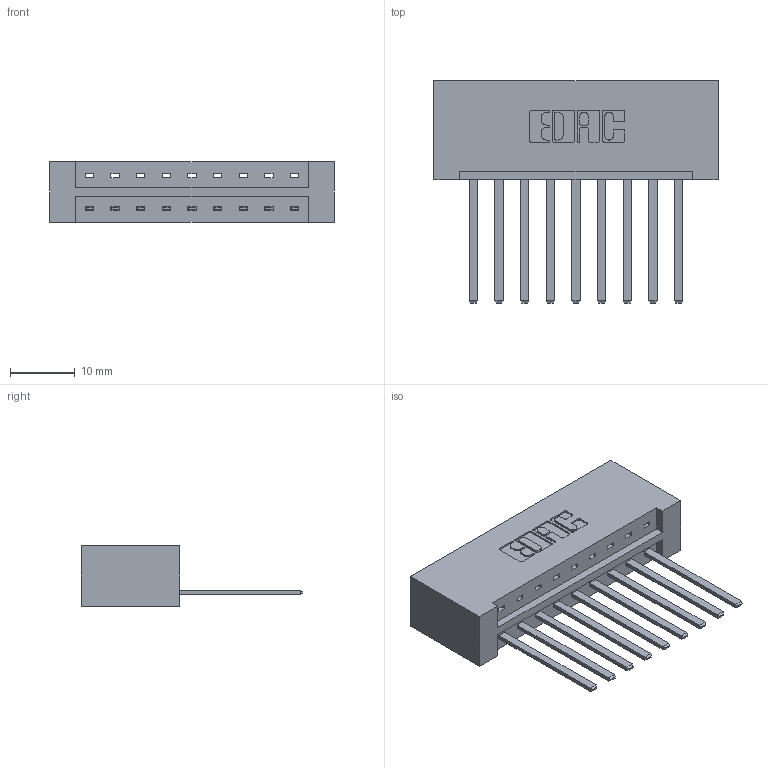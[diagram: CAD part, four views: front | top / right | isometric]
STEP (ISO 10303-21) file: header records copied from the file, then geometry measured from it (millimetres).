
FILE_DESCRIPTION (( 'STEP AP203' ), '1' );
FILE_NAME ('833-009-544-101.STEP', '2020-05-30T17:36:58', ( '' ), ( '' ), 'SwSTEP 2.0', 'SolidWorks 2020', '' );
FILE_SCHEMA (( 'CONFIG_CONTROL_DESIGN' ));
Length unit declared in the file: inch
Products named in the file (3): 833-009-544-101; 345-292-001_345-293-144; 833 Part_Lugless
Assembly tree (10 placements, depth 2):
  833-009-544-101
    833 Part_Lugless
    345-292-001_345-293-144  x9
Bounding box: 43.92 x 34.3 x 9.4 mm (x, y, z)
Volume: 4852.4 mm3; surface area: 5329.7 mm2
Topology: 10 solids, 10 shells, 574 faces, 1709 edges, 1126 vertices
Faces by surface type: plane 408, cylinder 166
Entity records: 9309 total; most frequent: CARTESIAN_POINT 1617, ORIENTED_EDGE 1562, DIRECTION 1419, EDGE_CURVE 781, LINE 665, VECTOR 665, VERTEX_POINT 518, AXIS2_PLACEMENT_3D 377
